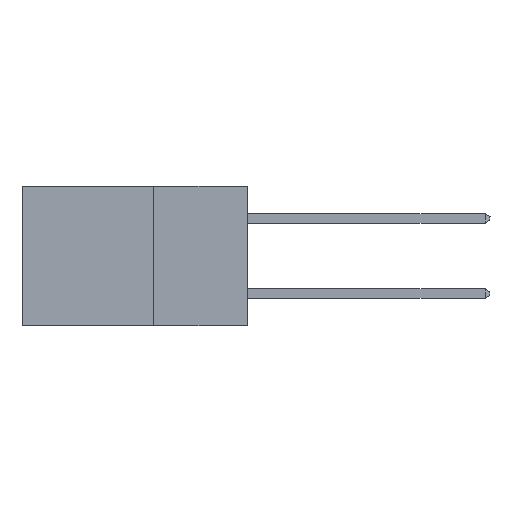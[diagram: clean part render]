
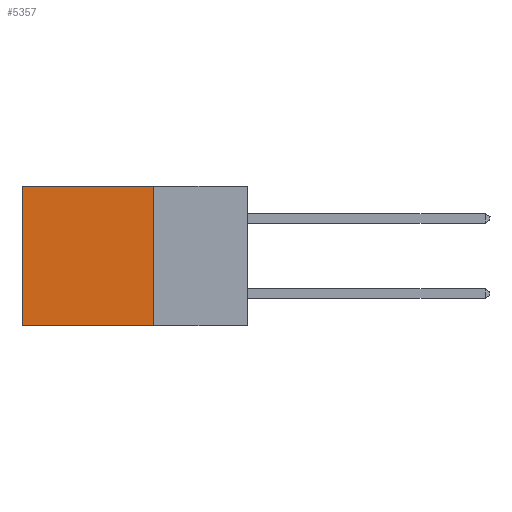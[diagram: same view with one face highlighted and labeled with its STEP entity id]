
A CAD part, left-side view. The second image highlights one B-rep face of the part: STEP entity #5357.
In plain terms, the highlighted planar face has unit normal (-1, 0, 0).
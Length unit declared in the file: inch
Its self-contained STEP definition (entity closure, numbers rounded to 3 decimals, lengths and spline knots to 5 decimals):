
#703 = ORIENTED_EDGE ( 'NONE', *, *, #15272, .F. ) ;
#1260 = EDGE_CURVE ( 'NONE', #4827, #4129, #12915, .T. ) ;
#2712 = DIRECTION ( 'NONE',  ( 1., 0., 0. ) ) ;
#2846 = LINE ( 'NONE', #4561, #6552 ) ;
#4129 = VERTEX_POINT ( 'NONE', #16652 ) ;
#4446 = DIRECTION ( 'NONE',  ( 0., 0., -1. ) ) ;
#4561 = CARTESIAN_POINT ( 'NONE',  ( 0.2615, 0.25, -0.37 ) ) ;
#4827 = VERTEX_POINT ( 'NONE', #19772 ) ;
#5357 = ADVANCED_FACE ( 'NONE', ( #25142 ), #14750, .F. ) ;
#6552 = VECTOR ( 'NONE', #6826, 39.37008 ) ;
#6826 = DIRECTION ( 'NONE',  ( 0., 1., 0. ) ) ;
#6865 = EDGE_LOOP ( 'NONE', ( #25711, #11803, #703, #8819 ) ) ;
#8819 = ORIENTED_EDGE ( 'NONE', *, *, #21203, .T. ) ;
#9659 = VECTOR ( 'NONE', #4446, 39.37008 ) ;
#9830 = LINE ( 'NONE', #20427, #19513 ) ;
#9846 = LINE ( 'NONE', #26047, #19684 ) ;
#10332 = DIRECTION ( 'NONE',  ( 0., 0., -1. ) ) ;
#10775 = DIRECTION ( 'NONE',  ( 0., 0., -1. ) ) ;
#10802 = CARTESIAN_POINT ( 'NONE',  ( 0.2615, 0.6, -0.37 ) ) ;
#11803 = ORIENTED_EDGE ( 'NONE', *, *, #23843, .F. ) ;
#12915 = LINE ( 'NONE', #10802, #9659 ) ;
#14750 = PLANE ( 'NONE',  #25871 ) ;
#15272 = EDGE_CURVE ( 'NONE', #22744, #18156, #9830, .T. ) ;
#16652 = CARTESIAN_POINT ( 'NONE',  ( 0.2615, 0.6, -0.37 ) ) ;
#18068 = CARTESIAN_POINT ( 'NONE',  ( 0.2615, 0.25, 0. ) ) ;
#18156 = VERTEX_POINT ( 'NONE', #18515 ) ;
#18515 = CARTESIAN_POINT ( 'NONE',  ( 0.2615, 0.25, -0.37 ) ) ;
#19144 = CARTESIAN_POINT ( 'NONE',  ( 0.2615, 0.25, -0.37 ) ) ;
#19513 = VECTOR ( 'NONE', #10332, 39.37008 ) ;
#19684 = VECTOR ( 'NONE', #25662, 39.37008 ) ;
#19772 = CARTESIAN_POINT ( 'NONE',  ( 0.2615, 0.6, 0. ) ) ;
#20427 = CARTESIAN_POINT ( 'NONE',  ( 0.2615, 0.25, -0.37 ) ) ;
#21203 = EDGE_CURVE ( 'NONE', #22744, #4827, #9846, .T. ) ;
#22744 = VERTEX_POINT ( 'NONE', #18068 ) ;
#23843 = EDGE_CURVE ( 'NONE', #18156, #4129, #2846, .T. ) ;
#25142 = FACE_OUTER_BOUND ( 'NONE', #6865, .T. ) ;
#25662 = DIRECTION ( 'NONE',  ( 0., 1., 0. ) ) ;
#25711 = ORIENTED_EDGE ( 'NONE', *, *, #1260, .T. ) ;
#25871 = AXIS2_PLACEMENT_3D ( 'NONE', #19144, #2712, #10775 ) ;
#26047 = CARTESIAN_POINT ( 'NONE',  ( 0.2615, 0.25, 0. ) ) ;
